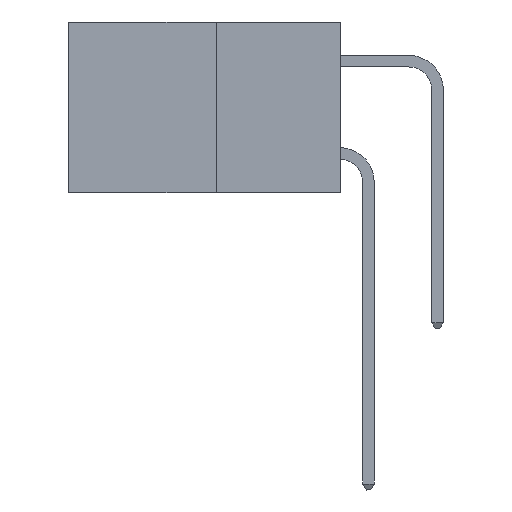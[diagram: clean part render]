
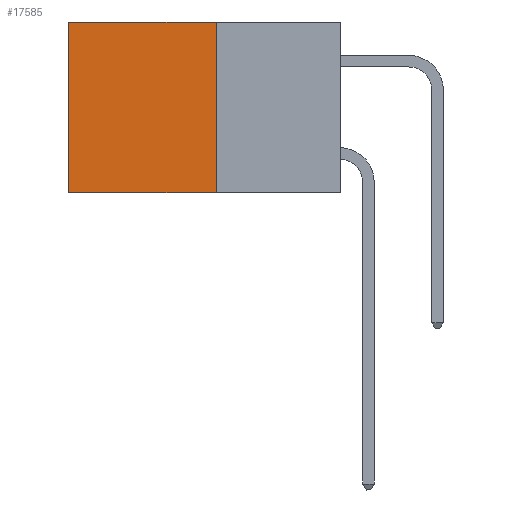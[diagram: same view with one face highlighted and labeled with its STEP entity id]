
A CAD part, left-side view. The second image highlights one B-rep face of the part: STEP entity #17585.
In plain terms, the highlighted planar face has unit normal (-1, 0, 0).
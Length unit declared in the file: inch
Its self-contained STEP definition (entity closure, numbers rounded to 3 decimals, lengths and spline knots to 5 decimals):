
#369 = CARTESIAN_POINT ( 'NONE',  ( 0.277, 0.27, 0. ) ) ;
#906 = VECTOR ( 'NONE', #8148, 39.37008 ) ;
#1184 = EDGE_LOOP ( 'NONE', ( #13975, #3190, #14761, #30925 ) ) ;
#1257 = EDGE_CURVE ( 'NONE', #5032, #2877, #14796, .T. ) ;
#1891 = CARTESIAN_POINT ( 'NONE',  ( 0.277, 0.59, -0.37 ) ) ;
#2309 = CARTESIAN_POINT ( 'NONE',  ( 0.277, 0.27, -0.37 ) ) ;
#2877 = VERTEX_POINT ( 'NONE', #20577 ) ;
#3190 = ORIENTED_EDGE ( 'NONE', *, *, #14148, .F. ) ;
#4882 = DIRECTION ( 'NONE',  ( 0., 0., -1. ) ) ;
#5032 = VERTEX_POINT ( 'NONE', #369 ) ;
#5264 = LINE ( 'NONE', #1891, #24343 ) ;
#6296 = VERTEX_POINT ( 'NONE', #28079 ) ;
#8008 = CARTESIAN_POINT ( 'NONE',  ( 0.277, 0.27, -0.37 ) ) ;
#8148 = DIRECTION ( 'NONE',  ( 0., 1., 0. ) ) ;
#8421 = VECTOR ( 'NONE', #26141, 39.37008 ) ;
#12618 = VERTEX_POINT ( 'NONE', #19533 ) ;
#12634 = PLANE ( 'NONE',  #31059 ) ;
#13975 = ORIENTED_EDGE ( 'NONE', *, *, #30806, .T. ) ;
#14148 = EDGE_CURVE ( 'NONE', #6296, #12618, #28469, .T. ) ;
#14761 = ORIENTED_EDGE ( 'NONE', *, *, #16797, .F. ) ;
#14796 = LINE ( 'NONE', #27408, #20071 ) ;
#16797 = EDGE_CURVE ( 'NONE', #5032, #6296, #22212, .T. ) ;
#17585 = ADVANCED_FACE ( 'NONE', ( #19001 ), #12634, .F. ) ;
#19001 = FACE_OUTER_BOUND ( 'NONE', #1184, .T. ) ;
#19533 = CARTESIAN_POINT ( 'NONE',  ( 0.277, 0.59, -0.37 ) ) ;
#20071 = VECTOR ( 'NONE', #29332, 39.37008 ) ;
#20458 = DIRECTION ( 'NONE',  ( 1., 0., 0. ) ) ;
#20577 = CARTESIAN_POINT ( 'NONE',  ( 0.277, 0.59, 0. ) ) ;
#22212 = LINE ( 'NONE', #8008, #8421 ) ;
#22621 = DIRECTION ( 'NONE',  ( 0., 0., -1. ) ) ;
#24343 = VECTOR ( 'NONE', #22621, 39.37008 ) ;
#26141 = DIRECTION ( 'NONE',  ( 0., 0., -1. ) ) ;
#27408 = CARTESIAN_POINT ( 'NONE',  ( 0.277, 0.27, 0. ) ) ;
#28079 = CARTESIAN_POINT ( 'NONE',  ( 0.277, 0.27, -0.37 ) ) ;
#28469 = LINE ( 'NONE', #28778, #906 ) ;
#28778 = CARTESIAN_POINT ( 'NONE',  ( 0.277, 0.27, -0.37 ) ) ;
#29332 = DIRECTION ( 'NONE',  ( 0., 1., 0. ) ) ;
#30806 = EDGE_CURVE ( 'NONE', #2877, #12618, #5264, .T. ) ;
#30925 = ORIENTED_EDGE ( 'NONE', *, *, #1257, .T. ) ;
#31059 = AXIS2_PLACEMENT_3D ( 'NONE', #2309, #20458, #4882 ) ;
